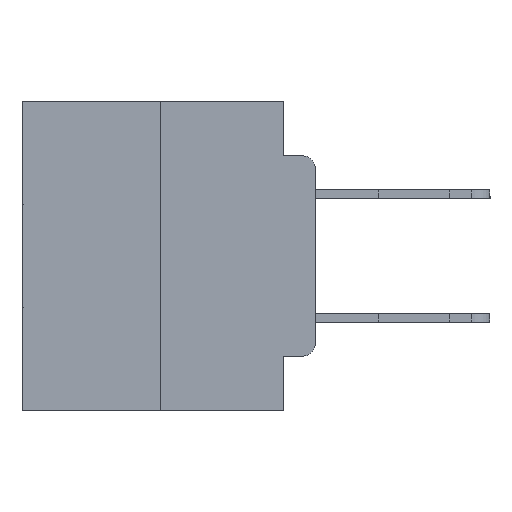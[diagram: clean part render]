
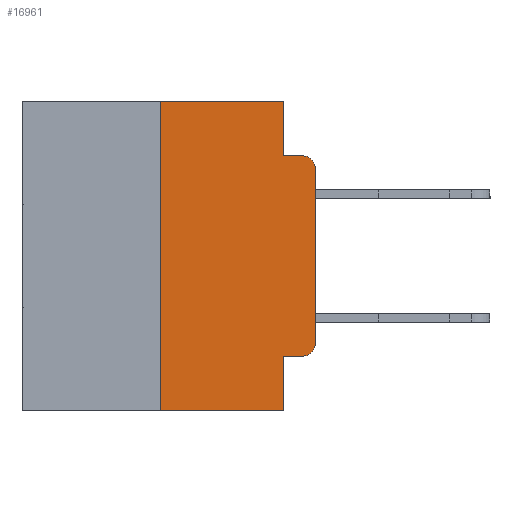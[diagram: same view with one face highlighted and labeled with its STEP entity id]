
A CAD part, left-side view. The second image highlights one B-rep face of the part: STEP entity #16961.
In plain terms, the highlighted planar face has unit normal (-1, 0, 0).
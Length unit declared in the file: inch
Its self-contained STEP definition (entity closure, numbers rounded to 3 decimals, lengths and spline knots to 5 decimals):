
#802 = LINE ( 'NONE', #15656, #12243 ) ;
#873 = VECTOR ( 'NONE', #26014, 39.37008 ) ;
#1058 = CARTESIAN_POINT ( 'NONE',  ( 0., 0.051, 0. ) ) ;
#1096 = CARTESIAN_POINT ( 'NONE',  ( 0., 0.02, -0.3915 ) ) ;
#2171 = EDGE_CURVE ( 'NONE', #9721, #2993, #7063, .T. ) ;
#2198 = CARTESIAN_POINT ( 'NONE',  ( 0., 0.25, 0. ) ) ;
#2790 = ORIENTED_EDGE ( 'NONE', *, *, #15295, .T. ) ;
#2993 = VERTEX_POINT ( 'NONE', #21155 ) ;
#3179 = LINE ( 'NONE', #11600, #26851 ) ;
#3227 = VERTEX_POINT ( 'NONE', #6347 ) ;
#3480 = CARTESIAN_POINT ( 'NONE',  ( 0., 0., 0. ) ) ;
#3486 = DIRECTION ( 'NONE',  ( 0., 0., -1. ) ) ;
#4019 = AXIS2_PLACEMENT_3D ( 'NONE', #18122, #4674, #20322 ) ;
#4589 = CARTESIAN_POINT ( 'NONE',  ( 0., 0.051, 0. ) ) ;
#4593 = VECTOR ( 'NONE', #25770, 39.37008 ) ;
#4674 = DIRECTION ( 'NONE',  ( -1., 0., 0. ) ) ;
#5001 = CIRCLE ( 'NONE', #4019, 0.02 ) ;
#5095 = CARTESIAN_POINT ( 'NONE',  ( 0., 0.473, 0. ) ) ;
#5507 = CARTESIAN_POINT ( 'NONE',  ( 0., 0.051, -0.4115 ) ) ;
#5800 = VERTEX_POINT ( 'NONE', #23959 ) ;
#6261 = VERTEX_POINT ( 'NONE', #25524 ) ;
#6330 = VERTEX_POINT ( 'NONE', #27840 ) ;
#6347 = CARTESIAN_POINT ( 'NONE',  ( 0., 0.051, 0. ) ) ;
#7063 = LINE ( 'NONE', #11627, #873 ) ;
#7419 = DIRECTION ( 'NONE',  ( 0., 0., -1. ) ) ;
#8199 = ORIENTED_EDGE ( 'NONE', *, *, #9314, .T. ) ;
#8524 = CIRCLE ( 'NONE', #17249, 0.02 ) ;
#9054 = DIRECTION ( 'NONE',  ( 0., 0., 1. ) ) ;
#9314 = EDGE_CURVE ( 'NONE', #23257, #16093, #5001, .T. ) ;
#9410 = LINE ( 'NONE', #1058, #16724 ) ;
#9721 = VERTEX_POINT ( 'NONE', #25606 ) ;
#10603 = LINE ( 'NONE', #3480, #4593 ) ;
#10778 = EDGE_CURVE ( 'NONE', #5800, #16093, #23735, .T. ) ;
#10986 = ORIENTED_EDGE ( 'NONE', *, *, #2171, .T. ) ;
#11487 = VERTEX_POINT ( 'NONE', #5507 ) ;
#11600 = CARTESIAN_POINT ( 'NONE',  ( 0., 0.473, 0. ) ) ;
#11627 = CARTESIAN_POINT ( 'NONE',  ( 0., 0.473, -0.5 ) ) ;
#11764 = VERTEX_POINT ( 'NONE', #15544 ) ;
#12243 = VECTOR ( 'NONE', #13386, 39.37008 ) ;
#12377 = ORIENTED_EDGE ( 'NONE', *, *, #16778, .T. ) ;
#12792 = VECTOR ( 'NONE', #20237, 39.37008 ) ;
#13386 = DIRECTION ( 'NONE',  ( 0., -1., 0. ) ) ;
#13765 = EDGE_CURVE ( 'NONE', #9721, #6261, #27511, .T. ) ;
#14077 = PLANE ( 'NONE',  #17562 ) ;
#14153 = ORIENTED_EDGE ( 'NONE', *, *, #10778, .F. ) ;
#14516 = EDGE_CURVE ( 'NONE', #6261, #3227, #3179, .T. ) ;
#14713 = DIRECTION ( 'NONE',  ( 0., 0., -1. ) ) ;
#15295 = EDGE_CURVE ( 'NONE', #6330, #23257, #10603, .T. ) ;
#15544 = CARTESIAN_POINT ( 'NONE',  ( 0., 0.02, -0.4115 ) ) ;
#15568 = ORIENTED_EDGE ( 'NONE', *, *, #14516, .F. ) ;
#15656 = CARTESIAN_POINT ( 'NONE',  ( 0., 0.051, -0.4115 ) ) ;
#16093 = VERTEX_POINT ( 'NONE', #28264 ) ;
#16474 = CARTESIAN_POINT ( 'NONE',  ( 0., 0.051, -0.0885 ) ) ;
#16724 = VECTOR ( 'NONE', #14713, 39.37008 ) ;
#16778 = EDGE_CURVE ( 'NONE', #11487, #11764, #802, .T. ) ;
#16961 = ADVANCED_FACE ( 'NONE', ( #24369 ), #14077, .F. ) ;
#16988 = DIRECTION ( 'NONE',  ( -1., 0., 0. ) ) ;
#17249 = AXIS2_PLACEMENT_3D ( 'NONE', #1096, #16988, #3486 ) ;
#17562 = AXIS2_PLACEMENT_3D ( 'NONE', #5095, #20753, #7419 ) ;
#17935 = VECTOR ( 'NONE', #18773, 39.37008 ) ;
#18048 = CARTESIAN_POINT ( 'NONE',  ( 0., 0., -0.1085 ) ) ;
#18122 = CARTESIAN_POINT ( 'NONE',  ( 0., 0.02, -0.1085 ) ) ;
#18246 = EDGE_CURVE ( 'NONE', #3227, #5800, #9410, .T. ) ;
#18773 = DIRECTION ( 'NONE',  ( 0., -1., 0. ) ) ;
#19716 = EDGE_CURVE ( 'NONE', #11487, #2993, #24570, .T. ) ;
#20237 = DIRECTION ( 'NONE',  ( 0., 0., -1. ) ) ;
#20322 = DIRECTION ( 'NONE',  ( 0., 0., -1. ) ) ;
#20753 = DIRECTION ( 'NONE',  ( 1., 0., 0. ) ) ;
#21155 = CARTESIAN_POINT ( 'NONE',  ( 0., 0.051, -0.5 ) ) ;
#21211 = EDGE_CURVE ( 'NONE', #11764, #6330, #8524, .T. ) ;
#21785 = EDGE_LOOP ( 'NONE', ( #2790, #8199, #14153, #26510, #15568, #27832, #10986, #22777, #12377, #24172 ) ) ;
#22777 = ORIENTED_EDGE ( 'NONE', *, *, #19716, .F. ) ;
#23257 = VERTEX_POINT ( 'NONE', #18048 ) ;
#23735 = LINE ( 'NONE', #16474, #17935 ) ;
#23959 = CARTESIAN_POINT ( 'NONE',  ( 0., 0.051, -0.0885 ) ) ;
#24172 = ORIENTED_EDGE ( 'NONE', *, *, #21211, .T. ) ;
#24369 = FACE_OUTER_BOUND ( 'NONE', #21785, .T. ) ;
#24570 = LINE ( 'NONE', #4589, #12792 ) ;
#25524 = CARTESIAN_POINT ( 'NONE',  ( 0., 0.25, 0. ) ) ;
#25606 = CARTESIAN_POINT ( 'NONE',  ( 0., 0.25, -0.5 ) ) ;
#25770 = DIRECTION ( 'NONE',  ( 0., 0., 1. ) ) ;
#26014 = DIRECTION ( 'NONE',  ( 0., -1., 0. ) ) ;
#26510 = ORIENTED_EDGE ( 'NONE', *, *, #18246, .F. ) ;
#26843 = VECTOR ( 'NONE', #9054, 39.37008 ) ;
#26851 = VECTOR ( 'NONE', #27006, 39.37008 ) ;
#27006 = DIRECTION ( 'NONE',  ( 0., -1., 0. ) ) ;
#27511 = LINE ( 'NONE', #2198, #26843 ) ;
#27832 = ORIENTED_EDGE ( 'NONE', *, *, #13765, .F. ) ;
#27840 = CARTESIAN_POINT ( 'NONE',  ( 0., 0., -0.3915 ) ) ;
#28264 = CARTESIAN_POINT ( 'NONE',  ( 0., 0.02, -0.0885 ) ) ;
